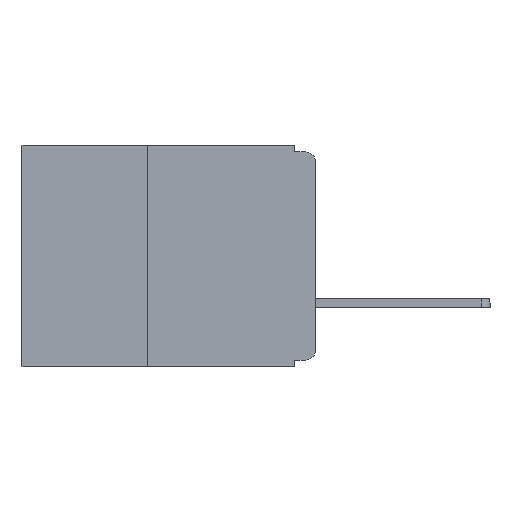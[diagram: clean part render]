
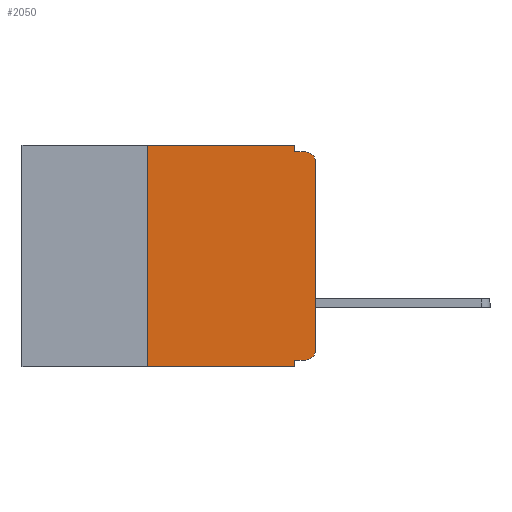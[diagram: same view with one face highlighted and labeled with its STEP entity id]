
A CAD part, left-side view. The second image highlights one B-rep face of the part: STEP entity #2050.
In plain terms, the highlighted planar face has unit normal (-1, 0, 0).
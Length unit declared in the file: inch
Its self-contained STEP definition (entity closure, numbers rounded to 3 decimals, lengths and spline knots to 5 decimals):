
#262 = VECTOR ( 'NONE', #24606, 39.37008 ) ;
#732 = CARTESIAN_POINT ( 'NONE',  ( 0., 0.031, 0. ) ) ;
#2050 = ADVANCED_FACE ( 'NONE', ( #19048 ), #28817, .F. ) ;
#2482 = ORIENTED_EDGE ( 'NONE', *, *, #29174, .F. ) ;
#3227 = VERTEX_POINT ( 'NONE', #26447 ) ;
#4880 = CARTESIAN_POINT ( 'NONE',  ( 0., 0.031, -0.33 ) ) ;
#4965 = CARTESIAN_POINT ( 'NONE',  ( 0., 0., -0.01 ) ) ;
#4997 = CARTESIAN_POINT ( 'NONE',  ( 0., 0.25, -0.33 ) ) ;
#5263 = EDGE_CURVE ( 'NONE', #16644, #3227, #7637, .T. ) ;
#5330 = CARTESIAN_POINT ( 'NONE',  ( 0., 0.031, -0.33 ) ) ;
#5568 = LINE ( 'NONE', #4997, #30924 ) ;
#5629 = EDGE_CURVE ( 'NONE', #14916, #9141, #11990, .T. ) ;
#6125 = ORIENTED_EDGE ( 'NONE', *, *, #5263, .F. ) ;
#6446 = LINE ( 'NONE', #4965, #12358 ) ;
#6631 = DIRECTION ( 'NONE',  ( -1., 0., 0. ) ) ;
#7002 = CIRCLE ( 'NONE', #21254, 0.015 ) ;
#7637 = LINE ( 'NONE', #24483, #19963 ) ;
#8190 = EDGE_CURVE ( 'NONE', #25597, #9537, #5568, .T. ) ;
#9141 = VERTEX_POINT ( 'NONE', #21038 ) ;
#9537 = VERTEX_POINT ( 'NONE', #22751 ) ;
#9830 = DIRECTION ( 'NONE',  ( -1., 0., 0. ) ) ;
#10053 = LINE ( 'NONE', #28392, #28818 ) ;
#10913 = LINE ( 'NONE', #20441, #23911 ) ;
#11236 = EDGE_CURVE ( 'NONE', #3227, #15770, #27299, .T. ) ;
#11990 = LINE ( 'NONE', #17720, #17722 ) ;
#12252 = EDGE_CURVE ( 'NONE', #25597, #15770, #10053, .T. ) ;
#12273 = CIRCLE ( 'NONE', #28973, 0.015 ) ;
#12358 = VECTOR ( 'NONE', #27128, 39.37008 ) ;
#13734 = ORIENTED_EDGE ( 'NONE', *, *, #5629, .T. ) ;
#13789 = DIRECTION ( 'NONE',  ( 0., -1., 0. ) ) ;
#14120 = AXIS2_PLACEMENT_3D ( 'NONE', #27840, #26081, #25516 ) ;
#14639 = CARTESIAN_POINT ( 'NONE',  ( 0., 0.25, -0.33 ) ) ;
#14916 = VERTEX_POINT ( 'NONE', #31004 ) ;
#15770 = VERTEX_POINT ( 'NONE', #5330 ) ;
#15867 = EDGE_CURVE ( 'NONE', #24743, #22269, #23333, .T. ) ;
#16105 = EDGE_CURVE ( 'NONE', #16644, #14916, #12273, .T. ) ;
#16644 = VERTEX_POINT ( 'NONE', #28434 ) ;
#16876 = VECTOR ( 'NONE', #20581, 39.37008 ) ;
#17313 = CARTESIAN_POINT ( 'NONE',  ( 0., 0.015, -0.01 ) ) ;
#17684 = DIRECTION ( 'NONE',  ( 0., 0., 1. ) ) ;
#17720 = CARTESIAN_POINT ( 'NONE',  ( 0., 0., 0. ) ) ;
#17722 = VECTOR ( 'NONE', #17684, 39.37008 ) ;
#18820 = EDGE_CURVE ( 'NONE', #9141, #25010, #7002, .T. ) ;
#18994 = EDGE_LOOP ( 'NONE', ( #13734, #24241, #19474, #26352, #2482, #23534, #28524, #22410, #6125, #24378 ) ) ;
#19048 = FACE_OUTER_BOUND ( 'NONE', #18994, .T. ) ;
#19474 = ORIENTED_EDGE ( 'NONE', *, *, #31376, .F. ) ;
#19963 = VECTOR ( 'NONE', #24159, 39.37008 ) ;
#20441 = CARTESIAN_POINT ( 'NONE',  ( 0., 0.437, 0. ) ) ;
#20581 = DIRECTION ( 'NONE',  ( 0., 0., -1. ) ) ;
#21038 = CARTESIAN_POINT ( 'NONE',  ( 0., 0., -0.025 ) ) ;
#21254 = AXIS2_PLACEMENT_3D ( 'NONE', #24516, #9830, #26963 ) ;
#21398 = CARTESIAN_POINT ( 'NONE',  ( 0., 0.015, -0.305 ) ) ;
#22241 = DIRECTION ( 'NONE',  ( 0., 0., 1. ) ) ;
#22269 = VERTEX_POINT ( 'NONE', #24680 ) ;
#22410 = ORIENTED_EDGE ( 'NONE', *, *, #11236, .F. ) ;
#22751 = CARTESIAN_POINT ( 'NONE',  ( 0., 0.25, 0. ) ) ;
#23333 = LINE ( 'NONE', #732, #16876 ) ;
#23502 = CARTESIAN_POINT ( 'NONE',  ( 0., 0.031, 0. ) ) ;
#23534 = ORIENTED_EDGE ( 'NONE', *, *, #8190, .F. ) ;
#23870 = DIRECTION ( 'NONE',  ( 0., 0., -1. ) ) ;
#23911 = VECTOR ( 'NONE', #30221, 39.37008 ) ;
#24159 = DIRECTION ( 'NONE',  ( 0., 1., 0. ) ) ;
#24241 = ORIENTED_EDGE ( 'NONE', *, *, #18820, .T. ) ;
#24378 = ORIENTED_EDGE ( 'NONE', *, *, #16105, .T. ) ;
#24483 = CARTESIAN_POINT ( 'NONE',  ( 0., 0., -0.32 ) ) ;
#24516 = CARTESIAN_POINT ( 'NONE',  ( 0., 0.015, -0.025 ) ) ;
#24606 = DIRECTION ( 'NONE',  ( 0., 0., -1. ) ) ;
#24680 = CARTESIAN_POINT ( 'NONE',  ( 0., 0.031, -0.01 ) ) ;
#24743 = VERTEX_POINT ( 'NONE', #23502 ) ;
#25010 = VERTEX_POINT ( 'NONE', #17313 ) ;
#25516 = DIRECTION ( 'NONE',  ( 0., 0., -1. ) ) ;
#25597 = VERTEX_POINT ( 'NONE', #14639 ) ;
#26081 = DIRECTION ( 'NONE',  ( 1., 0., 0. ) ) ;
#26352 = ORIENTED_EDGE ( 'NONE', *, *, #15867, .F. ) ;
#26447 = CARTESIAN_POINT ( 'NONE',  ( 0., 0.031, -0.32 ) ) ;
#26963 = DIRECTION ( 'NONE',  ( 0., 0., -1. ) ) ;
#27128 = DIRECTION ( 'NONE',  ( 0., -1., 0. ) ) ;
#27299 = LINE ( 'NONE', #4880, #262 ) ;
#27840 = CARTESIAN_POINT ( 'NONE',  ( 0., 0.437, 0. ) ) ;
#28392 = CARTESIAN_POINT ( 'NONE',  ( 0., 0.437, -0.33 ) ) ;
#28434 = CARTESIAN_POINT ( 'NONE',  ( 0., 0.015, -0.32 ) ) ;
#28524 = ORIENTED_EDGE ( 'NONE', *, *, #12252, .T. ) ;
#28817 = PLANE ( 'NONE',  #14120 ) ;
#28818 = VECTOR ( 'NONE', #13789, 39.37008 ) ;
#28973 = AXIS2_PLACEMENT_3D ( 'NONE', #21398, #6631, #23870 ) ;
#29174 = EDGE_CURVE ( 'NONE', #9537, #24743, #10913, .T. ) ;
#30221 = DIRECTION ( 'NONE',  ( 0., -1., 0. ) ) ;
#30924 = VECTOR ( 'NONE', #22241, 39.37008 ) ;
#31004 = CARTESIAN_POINT ( 'NONE',  ( 0., 0., -0.305 ) ) ;
#31376 = EDGE_CURVE ( 'NONE', #22269, #25010, #6446, .T. ) ;
